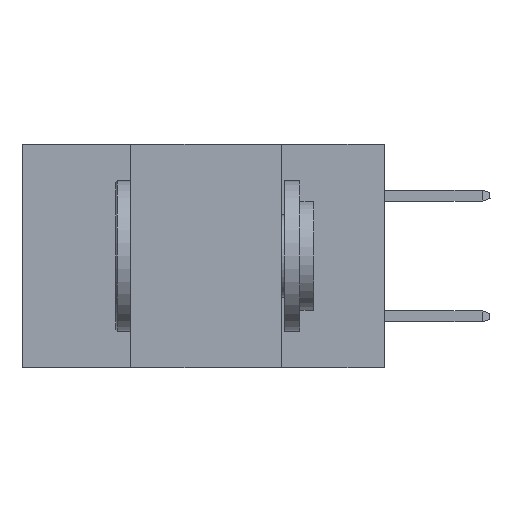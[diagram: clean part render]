
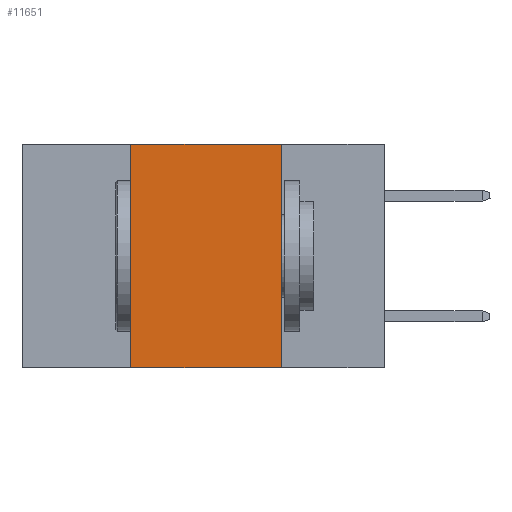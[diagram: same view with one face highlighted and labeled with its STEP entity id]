
A CAD part, left-side view. The second image highlights one B-rep face of the part: STEP entity #11651.
In plain terms, the highlighted planar face has unit normal (-1, 0, 0).
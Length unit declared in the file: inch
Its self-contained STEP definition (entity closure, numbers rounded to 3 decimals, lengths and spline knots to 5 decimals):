
#160 = LINE ( 'NONE', #7619, #843 ) ;
#821 = EDGE_CURVE ( 'NONE', #8872, #10939, #17195, .T. ) ;
#843 = VECTOR ( 'NONE', #15924, 39.37008 ) ;
#1119 = DIRECTION ( 'NONE',  ( 0., 0., -1. ) ) ;
#1209 = PLANE ( 'NONE',  #7145 ) ;
#1755 = CARTESIAN_POINT ( 'NONE',  ( 0., 0.42, 0. ) ) ;
#2350 = VERTEX_POINT ( 'NONE', #16455 ) ;
#3610 = ORIENTED_EDGE ( 'NONE', *, *, #13904, .T. ) ;
#5290 = FACE_OUTER_BOUND ( 'NONE', #12753, .T. ) ;
#5578 = LINE ( 'NONE', #1755, #15316 ) ;
#5729 = VECTOR ( 'NONE', #1119, 39.37008 ) ;
#5935 = DIRECTION ( 'NONE',  ( 0., 0., 1. ) ) ;
#6233 = ORIENTED_EDGE ( 'NONE', *, *, #821, .F. ) ;
#7080 = CARTESIAN_POINT ( 'NONE',  ( 0., 0.42, -0.37 ) ) ;
#7145 = AXIS2_PLACEMENT_3D ( 'NONE', #9510, #10951, #7822 ) ;
#7619 = CARTESIAN_POINT ( 'NONE',  ( 0., 0.6, 0. ) ) ;
#7822 = DIRECTION ( 'NONE',  ( 0., 0., -1. ) ) ;
#8165 = CARTESIAN_POINT ( 'NONE',  ( 0., 0.17, 0. ) ) ;
#8610 = DIRECTION ( 'NONE',  ( 0., -1., 0. ) ) ;
#8872 = VERTEX_POINT ( 'NONE', #14093 ) ;
#9510 = CARTESIAN_POINT ( 'NONE',  ( 0., 0.6, 0. ) ) ;
#10229 = VECTOR ( 'NONE', #8610, 39.37008 ) ;
#10271 = EDGE_CURVE ( 'NONE', #14025, #2350, #5578, .T. ) ;
#10939 = VERTEX_POINT ( 'NONE', #16159 ) ;
#10951 = DIRECTION ( 'NONE',  ( 1., 0., 0. ) ) ;
#11651 = ADVANCED_FACE ( 'NONE', ( #5290 ), #1209, .F. ) ;
#12753 = EDGE_LOOP ( 'NONE', ( #6233, #15522, #13655, #3610 ) ) ;
#13588 = CARTESIAN_POINT ( 'NONE',  ( 0., 0.6, -0.37 ) ) ;
#13655 = ORIENTED_EDGE ( 'NONE', *, *, #10271, .F. ) ;
#13904 = EDGE_CURVE ( 'NONE', #14025, #10939, #15179, .T. ) ;
#14025 = VERTEX_POINT ( 'NONE', #7080 ) ;
#14093 = CARTESIAN_POINT ( 'NONE',  ( 0., 0.17, 0. ) ) ;
#15112 = EDGE_CURVE ( 'NONE', #2350, #8872, #160, .T. ) ;
#15179 = LINE ( 'NONE', #13588, #10229 ) ;
#15316 = VECTOR ( 'NONE', #5935, 39.37008 ) ;
#15522 = ORIENTED_EDGE ( 'NONE', *, *, #15112, .F. ) ;
#15924 = DIRECTION ( 'NONE',  ( 0., -1., 0. ) ) ;
#16159 = CARTESIAN_POINT ( 'NONE',  ( 0., 0.17, -0.37 ) ) ;
#16455 = CARTESIAN_POINT ( 'NONE',  ( 0., 0.42, 0. ) ) ;
#17195 = LINE ( 'NONE', #8165, #5729 ) ;
